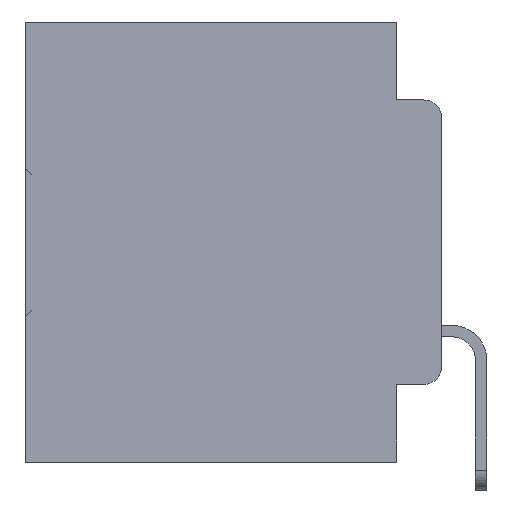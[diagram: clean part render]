
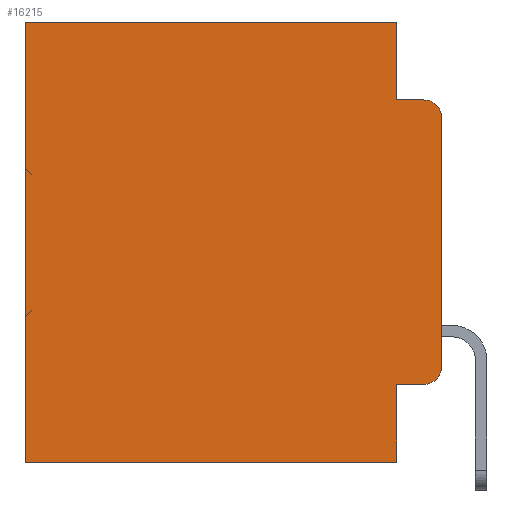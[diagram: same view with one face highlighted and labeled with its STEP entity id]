
A CAD part, left-side view. The second image highlights one B-rep face of the part: STEP entity #16215.
In plain terms, the highlighted planar face has unit normal (-1, 0, 0).
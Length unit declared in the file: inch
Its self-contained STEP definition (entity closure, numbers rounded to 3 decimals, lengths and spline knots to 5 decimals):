
#623 = DIRECTION ( 'NONE',  ( -1., 0., 0. ) ) ;
#871 = PLANE ( 'NONE',  #31433 ) ;
#988 = VERTEX_POINT ( 'NONE', #17765 ) ;
#1644 = EDGE_CURVE ( 'NONE', #10800, #988, #4676, .T. ) ;
#2474 = DIRECTION ( 'NONE',  ( 0., 0., -1. ) ) ;
#3028 = CARTESIAN_POINT ( 'NONE',  ( 0.298, 0.02, -0.4115 ) ) ;
#3066 = EDGE_CURVE ( 'NONE', #24878, #17973, #11777, .T. ) ;
#3323 = CIRCLE ( 'NONE', #31900, 0.02 ) ;
#3748 = VECTOR ( 'NONE', #26877, 39.37008 ) ;
#3838 = DIRECTION ( 'NONE',  ( 0., 0., -1. ) ) ;
#3982 = DIRECTION ( 'NONE',  ( 0., 1., 0. ) ) ;
#4042 = VECTOR ( 'NONE', #8676, 39.37008 ) ;
#4656 = AXIS2_PLACEMENT_3D ( 'NONE', #17779, #623, #20568 ) ;
#4676 = LINE ( 'NONE', #27642, #3748 ) ;
#5408 = VERTEX_POINT ( 'NONE', #26162 ) ;
#5734 = CARTESIAN_POINT ( 'NONE',  ( 0.298, 0.051, -0.4115 ) ) ;
#6912 = CIRCLE ( 'NONE', #4656, 0.02 ) ;
#7090 = LINE ( 'NONE', #31528, #14618 ) ;
#7131 = EDGE_CURVE ( 'NONE', #31955, #35840, #3323, .T. ) ;
#8566 = EDGE_LOOP ( 'NONE', ( #15980, #36305, #26195, #30080, #12186, #10019, #23181, #17082, #30052, #35653 ) ) ;
#8676 = DIRECTION ( 'NONE',  ( 0., 0., -1. ) ) ;
#10019 = ORIENTED_EDGE ( 'NONE', *, *, #21807, .T. ) ;
#10479 = VERTEX_POINT ( 'NONE', #29667 ) ;
#10673 = CARTESIAN_POINT ( 'NONE',  ( 0.298, 0.473, -0.5 ) ) ;
#10800 = VERTEX_POINT ( 'NONE', #31118 ) ;
#11777 = LINE ( 'NONE', #33848, #24906 ) ;
#12077 = DIRECTION ( 'NONE',  ( 0., -1., 0. ) ) ;
#12186 = ORIENTED_EDGE ( 'NONE', *, *, #27269, .T. ) ;
#12613 = DIRECTION ( 'NONE',  ( 0., 0., -1. ) ) ;
#13084 = CARTESIAN_POINT ( 'NONE',  ( 0.298, 0., 0. ) ) ;
#14334 = VECTOR ( 'NONE', #3982, 39.37008 ) ;
#14618 = VECTOR ( 'NONE', #12077, 39.37008 ) ;
#14818 = CARTESIAN_POINT ( 'NONE',  ( 0.298, 0.02, -0.0885 ) ) ;
#15935 = DIRECTION ( 'NONE',  ( 0., 0., -1. ) ) ;
#15980 = ORIENTED_EDGE ( 'NONE', *, *, #18473, .F. ) ;
#16215 = ADVANCED_FACE ( 'NONE', ( #25061 ), #871, .F. ) ;
#17024 = DIRECTION ( 'NONE',  ( 0., -1., 0. ) ) ;
#17082 = ORIENTED_EDGE ( 'NONE', *, *, #24363, .F. ) ;
#17765 = CARTESIAN_POINT ( 'NONE',  ( 0.298, 0.051, -0.0885 ) ) ;
#17779 = CARTESIAN_POINT ( 'NONE',  ( 0.298, 0.02, -0.3915 ) ) ;
#17973 = VERTEX_POINT ( 'NONE', #10673 ) ;
#18012 = CARTESIAN_POINT ( 'NONE',  ( 0.298, 0., 0. ) ) ;
#18473 = EDGE_CURVE ( 'NONE', #31955, #5408, #20521, .T. ) ;
#18480 = LINE ( 'NONE', #33432, #20245 ) ;
#18766 = VECTOR ( 'NONE', #15935, 39.37008 ) ;
#19276 = VERTEX_POINT ( 'NONE', #3028 ) ;
#20245 = VECTOR ( 'NONE', #2474, 39.37008 ) ;
#20521 = LINE ( 'NONE', #13084, #18766 ) ;
#20568 = DIRECTION ( 'NONE',  ( 0., 0., -1. ) ) ;
#20817 = DIRECTION ( 'NONE',  ( 1., 0., 0. ) ) ;
#20914 = LINE ( 'NONE', #20954, #14334 ) ;
#20954 = CARTESIAN_POINT ( 'NONE',  ( 0.298, 0., 0. ) ) ;
#20976 = LINE ( 'NONE', #5734, #34780 ) ;
#21807 = EDGE_CURVE ( 'NONE', #28831, #17973, #18480, .T. ) ;
#23181 = ORIENTED_EDGE ( 'NONE', *, *, #3066, .F. ) ;
#24363 = EDGE_CURVE ( 'NONE', #10479, #24878, #33006, .T. ) ;
#24878 = VERTEX_POINT ( 'NONE', #31055 ) ;
#24906 = VECTOR ( 'NONE', #33774, 39.37008 ) ;
#25061 = FACE_OUTER_BOUND ( 'NONE', #8566, .T. ) ;
#25977 = EDGE_CURVE ( 'NONE', #19276, #5408, #6912, .T. ) ;
#26162 = CARTESIAN_POINT ( 'NONE',  ( 0.298, 0., -0.3915 ) ) ;
#26195 = ORIENTED_EDGE ( 'NONE', *, *, #32145, .F. ) ;
#26444 = EDGE_CURVE ( 'NONE', #10479, #19276, #20976, .T. ) ;
#26877 = DIRECTION ( 'NONE',  ( 0., 0., -1. ) ) ;
#27269 = EDGE_CURVE ( 'NONE', #10800, #28831, #20914, .T. ) ;
#27642 = CARTESIAN_POINT ( 'NONE',  ( 0.298, 0.051, 0. ) ) ;
#27858 = CARTESIAN_POINT ( 'NONE',  ( 0.298, 0.473, 0. ) ) ;
#28189 = CARTESIAN_POINT ( 'NONE',  ( 0.298, 0.051, 0. ) ) ;
#28831 = VERTEX_POINT ( 'NONE', #27858 ) ;
#29667 = CARTESIAN_POINT ( 'NONE',  ( 0.298, 0.051, -0.4115 ) ) ;
#30052 = ORIENTED_EDGE ( 'NONE', *, *, #26444, .T. ) ;
#30080 = ORIENTED_EDGE ( 'NONE', *, *, #1644, .F. ) ;
#31055 = CARTESIAN_POINT ( 'NONE',  ( 0.298, 0.051, -0.5 ) ) ;
#31118 = CARTESIAN_POINT ( 'NONE',  ( 0.298, 0.051, 0. ) ) ;
#31433 = AXIS2_PLACEMENT_3D ( 'NONE', #18012, #20817, #3838 ) ;
#31528 = CARTESIAN_POINT ( 'NONE',  ( 0.298, 0.051, -0.0885 ) ) ;
#31900 = AXIS2_PLACEMENT_3D ( 'NONE', #35040, #33056, #12613 ) ;
#31955 = VERTEX_POINT ( 'NONE', #36223 ) ;
#32145 = EDGE_CURVE ( 'NONE', #988, #35840, #7090, .T. ) ;
#33006 = LINE ( 'NONE', #28189, #4042 ) ;
#33056 = DIRECTION ( 'NONE',  ( -1., 0., 0. ) ) ;
#33432 = CARTESIAN_POINT ( 'NONE',  ( 0.298, 0.473, 0. ) ) ;
#33774 = DIRECTION ( 'NONE',  ( 0., 1., 0. ) ) ;
#33848 = CARTESIAN_POINT ( 'NONE',  ( 0.298, 0., -0.5 ) ) ;
#34780 = VECTOR ( 'NONE', #17024, 39.37008 ) ;
#35040 = CARTESIAN_POINT ( 'NONE',  ( 0.298, 0.02, -0.1085 ) ) ;
#35653 = ORIENTED_EDGE ( 'NONE', *, *, #25977, .T. ) ;
#35840 = VERTEX_POINT ( 'NONE', #14818 ) ;
#36223 = CARTESIAN_POINT ( 'NONE',  ( 0.298, 0., -0.1085 ) ) ;
#36305 = ORIENTED_EDGE ( 'NONE', *, *, #7131, .T. ) ;
